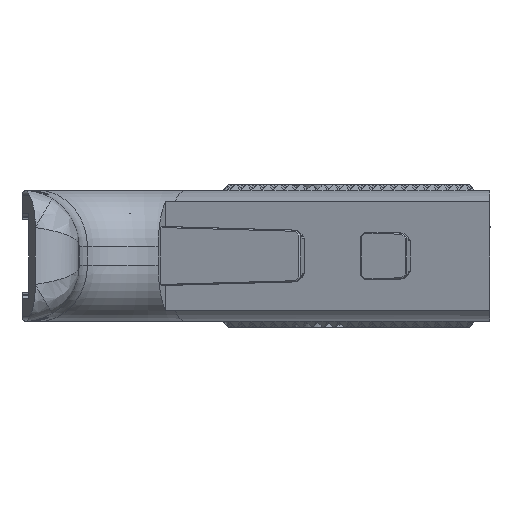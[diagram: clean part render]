
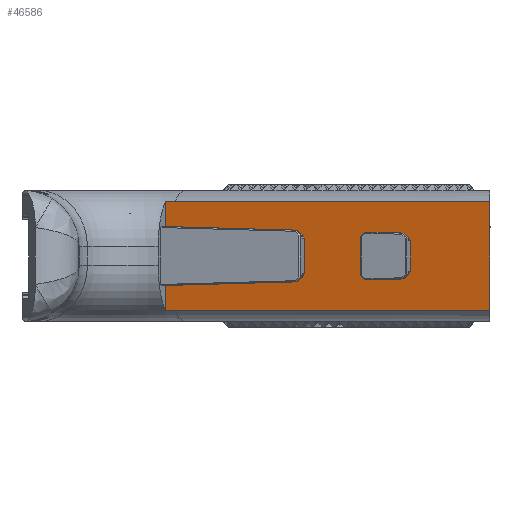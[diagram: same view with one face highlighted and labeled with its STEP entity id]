
A CAD part, left-side view. The second image highlights one B-rep face of the part: STEP entity #46586.
In plain terms, the highlighted planar face has unit normal (-0.951, 0.309, 0).
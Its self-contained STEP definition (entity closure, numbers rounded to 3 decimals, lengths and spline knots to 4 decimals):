
#2528=PLANE('',#49719);
#2773=FACE_BOUND('',#19868,.T.);
#7824=LINE('',#89198,#13351);
#7842=LINE('',#89236,#13369);
#7850=LINE('',#89253,#13377);
#7855=LINE('',#89262,#13382);
#7857=LINE('',#89265,#13384);
#7859=LINE('',#89270,#13386);
#7861=LINE('',#89274,#13388);
#7863=LINE('',#89277,#13390);
#7865=LINE('',#89281,#13392);
#7866=LINE('',#89283,#13393);
#7872=LINE('',#89296,#13399);
#7874=LINE('',#89300,#13401);
#7875=LINE('',#89303,#13402);
#7877=LINE('',#89307,#13404);
#7878=LINE('',#89317,#13405);
#7879=LINE('',#89319,#13406);
#7880=LINE('',#89321,#13407);
#7881=LINE('',#89331,#13408);
#7882=LINE('',#89332,#13409);
#13351=VECTOR('',#60471,0.3937);
#13369=VECTOR('',#60507,0.3937);
#13377=VECTOR('',#60521,0.3937);
#13382=VECTOR('',#60530,0.3937);
#13384=VECTOR('',#60534,0.3937);
#13386=VECTOR('',#60538,0.3937);
#13388=VECTOR('',#60542,0.3937);
#13390=VECTOR('',#60546,0.3937);
#13392=VECTOR('',#60550,0.3937);
#13393=VECTOR('',#60553,0.3937);
#13399=VECTOR('',#60569,0.3937);
#13401=VECTOR('',#60573,0.3937);
#13402=VECTOR('',#60576,0.3937);
#13404=VECTOR('',#60580,0.3937);
#13405=VECTOR('',#60581,0.3937);
#13406=VECTOR('',#60582,0.3937);
#13407=VECTOR('',#60583,0.3937);
#13408=VECTOR('',#60584,0.3937);
#13409=VECTOR('',#60585,0.3937);
#16849=FACE_OUTER_BOUND('',#19867,.T.);
#19867=EDGE_LOOP('',(#41645,#41646,#41647,#41648,#41649,#41650,#41651,#41652,
#41653,#41654,#41655,#41656));
#19868=EDGE_LOOP('',(#41657,#41658,#41659,#41660,#41661,#41662,#41663,#41664,
#41665));
#20883=B_SPLINE_CURVE_WITH_KNOTS('',3,(#89309,#89310,#89311,#89312,#89313,
#89314,#89315),.UNSPECIFIED.,.F.,.F.,(4,3,4),(0.,0.1181,0.2155),
 .UNSPECIFIED.);
#20884=B_SPLINE_CURVE_WITH_KNOTS('',3,(#89323,#89324,#89325,#89326,#89327,
#89328,#89329),.UNSPECIFIED.,.F.,.F.,(4,3,4),(-0.2155,-0.1181,
0.),.UNSPECIFIED.);
#23791=VERTEX_POINT('',#89195);
#23792=VERTEX_POINT('',#89197);
#23802=VERTEX_POINT('',#89233);
#23803=VERTEX_POINT('',#89235);
#23808=VERTEX_POINT('',#89250);
#23809=VERTEX_POINT('',#89252);
#23811=VERTEX_POINT('',#89261);
#23812=VERTEX_POINT('',#89267);
#23813=VERTEX_POINT('',#89269);
#23814=VERTEX_POINT('',#89273);
#23815=VERTEX_POINT('',#89279);
#23817=VERTEX_POINT('',#89294);
#23818=VERTEX_POINT('',#89298);
#23819=VERTEX_POINT('',#89302);
#23820=VERTEX_POINT('',#89306);
#23821=VERTEX_POINT('',#89308);
#23822=VERTEX_POINT('',#89316);
#23823=VERTEX_POINT('',#89318);
#23824=VERTEX_POINT('',#89320);
#23825=VERTEX_POINT('',#89322);
#23826=VERTEX_POINT('',#89330);
#29843=EDGE_CURVE('',#23792,#23791,#7824,.T.);
#29861=EDGE_CURVE('',#23802,#23803,#7842,.T.);
#29869=EDGE_CURVE('',#23808,#23809,#7850,.F.);
#29874=EDGE_CURVE('',#23792,#23811,#7855,.F.);
#29876=EDGE_CURVE('',#23808,#23811,#7857,.T.);
#29878=EDGE_CURVE('',#23812,#23813,#7859,.F.);
#29880=EDGE_CURVE('',#23814,#23813,#7861,.T.);
#29882=EDGE_CURVE('',#23812,#23809,#7863,.T.);
#29884=EDGE_CURVE('',#23815,#23791,#7865,.F.);
#29885=EDGE_CURVE('',#23814,#23815,#7866,.F.);
#29891=EDGE_CURVE('',#23817,#23802,#7872,.F.);
#29893=EDGE_CURVE('',#23817,#23818,#7874,.T.);
#29894=EDGE_CURVE('',#23803,#23819,#7875,.F.);
#29896=EDGE_CURVE('',#23820,#23818,#7877,.T.);
#29897=EDGE_CURVE('',#23821,#23820,#20883,.T.);
#29898=EDGE_CURVE('',#23822,#23821,#7878,.T.);
#29899=EDGE_CURVE('',#23823,#23822,#7879,.T.);
#29900=EDGE_CURVE('',#23824,#23823,#7880,.T.);
#29901=EDGE_CURVE('',#23825,#23824,#20884,.T.);
#29902=EDGE_CURVE('',#23826,#23825,#7881,.T.);
#29903=EDGE_CURVE('',#23826,#23819,#7882,.T.);
#41645=ORIENTED_EDGE('',*,*,#29893,.T.);
#41646=ORIENTED_EDGE('',*,*,#29896,.F.);
#41647=ORIENTED_EDGE('',*,*,#29897,.F.);
#41648=ORIENTED_EDGE('',*,*,#29898,.F.);
#41649=ORIENTED_EDGE('',*,*,#29899,.F.);
#41650=ORIENTED_EDGE('',*,*,#29900,.F.);
#41651=ORIENTED_EDGE('',*,*,#29901,.F.);
#41652=ORIENTED_EDGE('',*,*,#29902,.F.);
#41653=ORIENTED_EDGE('',*,*,#29903,.T.);
#41654=ORIENTED_EDGE('',*,*,#29894,.F.);
#41655=ORIENTED_EDGE('',*,*,#29861,.F.);
#41656=ORIENTED_EDGE('',*,*,#29891,.F.);
#41657=ORIENTED_EDGE('',*,*,#29843,.T.);
#41658=ORIENTED_EDGE('',*,*,#29884,.F.);
#41659=ORIENTED_EDGE('',*,*,#29885,.F.);
#41660=ORIENTED_EDGE('',*,*,#29880,.T.);
#41661=ORIENTED_EDGE('',*,*,#29878,.F.);
#41662=ORIENTED_EDGE('',*,*,#29882,.T.);
#41663=ORIENTED_EDGE('',*,*,#29869,.F.);
#41664=ORIENTED_EDGE('',*,*,#29876,.T.);
#41665=ORIENTED_EDGE('',*,*,#29874,.F.);
#46586=ADVANCED_FACE('',(#16849,#2773),#2528,.T.);
#49719=AXIS2_PLACEMENT_3D('',#89305,#60578,#60579);
#60471=DIRECTION('',(0.,0.,1.));
#60507=DIRECTION('',(0.,0.,1.));
#60521=DIRECTION('',(0.216,0.664,-0.716));
#60530=DIRECTION('',(0.221,0.681,0.698));
#60534=DIRECTION('',(0.309,0.951,-0.026));
#60538=DIRECTION('',(-0.216,-0.664,-0.716));
#60542=DIRECTION('',(-0.309,-0.951,-0.026));
#60546=DIRECTION('',(0.,0.,-1.));
#60550=DIRECTION('',(-0.12,-0.37,0.921));
#60553=DIRECTION('',(-0.221,-0.681,0.698));
#60569=DIRECTION('',(0.216,0.664,-0.716));
#60573=DIRECTION('',(0.309,0.951,-0.026));
#60576=DIRECTION('',(-0.216,-0.664,-0.716));
#60578=DIRECTION('center_axis',(-0.951,0.309,0.));
#60579=DIRECTION('ref_axis',(0.,0.,
1.));
#60580=DIRECTION('',(0.,0.,1.));
#60581=DIRECTION('',(0.309,0.951,0.));
#60582=DIRECTION('',(0.,0.,-1.));
#60583=DIRECTION('',(-0.309,-0.951,0.));
#60584=DIRECTION('',(0.,0.,1.));
#60585=DIRECTION('',(-0.309,-0.951,-0.026));
#89195=CARTESIAN_POINT('',(-2.8962,-0.8838,-0.6352));
#89197=CARTESIAN_POINT('',(-2.8962,-0.8838,-0.9101));
#89198=CARTESIAN_POINT('',(-2.8962,-0.8838,-0.7677));
#89233=CARTESIAN_POINT('',(-2.7262,-0.3607,-0.9245));
#89235=CARTESIAN_POINT('',(-2.7262,-0.3607,-0.6109));
#89236=CARTESIAN_POINT('',(-2.7262,-0.3607,-0.9154));
#89250=CARTESIAN_POINT('',(-3.0247,-1.2792,-0.909));
#89252=CARTESIAN_POINT('',(-3.0277,-1.2886,-0.8989));
#89253=CARTESIAN_POINT('',(-2.9908,-1.1749,-1.0217));
#89261=CARTESIAN_POINT('',(-2.8992,-0.8932,-0.9197));
#89262=CARTESIAN_POINT('',(-2.8709,-0.806,-0.8303));
#89265=CARTESIAN_POINT('',(-3.0469,-1.3476,-0.9072));
#89267=CARTESIAN_POINT('',(-3.0277,-1.2886,-0.6365));
#89269=CARTESIAN_POINT('',(-3.0247,-1.2792,-0.6264));
#89270=CARTESIAN_POINT('',(-2.9908,-1.1749,-0.5138));
#89273=CARTESIAN_POINT('',(-2.8992,-0.8932,-0.6158));
#89274=CARTESIAN_POINT('',(-3.0469,-1.3476,-0.6283));
#89277=CARTESIAN_POINT('',(-3.0277,-1.2886,-0.899));
#89279=CARTESIAN_POINT('',(-2.8984,-0.8905,-0.6185));
#89281=CARTESIAN_POINT('',(-2.885,-0.8493,-0.7213));
#89283=CARTESIAN_POINT('',(-2.8709,-0.806,-0.7051));
#89294=CARTESIAN_POINT('',(-2.7232,-0.3514,-0.9346));
#89296=CARTESIAN_POINT('',(-2.7647,-0.479,-0.7968));
#89298=CARTESIAN_POINT('',(-2.3324,0.8513,-0.9677));
#89300=CARTESIAN_POINT('',(-3.0469,-1.3476,-0.9072));
#89302=CARTESIAN_POINT('',(-2.7232,-0.3514,-0.6008));
#89303=CARTESIAN_POINT('',(-2.7647,-0.479,-0.7386));
#89305=CARTESIAN_POINT('Origin',(-2.8375,-0.7031,-0.7677));
#89306=CARTESIAN_POINT('',(-2.3324,0.8513,-1.2459));
#89307=CARTESIAN_POINT('',(-2.3324,0.8513,-1.0302));
#89308=CARTESIAN_POINT('',(-2.3592,0.7689,-1.2425));
#89309=CARTESIAN_POINT('Ctrl Pts',(-2.3592,0.7689,
-1.2425));
#89310=CARTESIAN_POINT('Ctrl Pts',(-2.3544,0.7836,
-1.2425));
#89311=CARTESIAN_POINT('Ctrl Pts',(-2.3495,0.7986,
-1.2428));
#89312=CARTESIAN_POINT('Ctrl Pts',(-2.3446,0.8138,
-1.2435));
#89313=CARTESIAN_POINT('Ctrl Pts',(-2.3405,0.8264,
-1.2441));
#89314=CARTESIAN_POINT('Ctrl Pts',(-2.3365,0.8388,
-1.2449));
#89315=CARTESIAN_POINT('Ctrl Pts',(-2.3324,0.8513,-1.2459));
#89316=CARTESIAN_POINT('',(-3.2516,-1.9775,-1.2425));
#89317=CARTESIAN_POINT('',(-2.1969,1.2684,-1.2425));
#89318=CARTESIAN_POINT('',(-3.2516,-1.9775,-0.2929));
#89319=CARTESIAN_POINT('',(-3.2516,-1.9775,-0.3839));
#89320=CARTESIAN_POINT('',(-2.3592,0.7689,-0.2929));
#89321=CARTESIAN_POINT('',(-2.6906,-0.2509,-0.2929));
#89322=CARTESIAN_POINT('',(-2.3324,0.8513,-0.2895));
#89323=CARTESIAN_POINT('Ctrl Pts',(-2.3324,0.8513,-0.2895));
#89324=CARTESIAN_POINT('Ctrl Pts',(-2.3365,0.8388,
-0.2905));
#89325=CARTESIAN_POINT('Ctrl Pts',(-2.3405,0.8264,
-0.2913));
#89326=CARTESIAN_POINT('Ctrl Pts',(-2.3446,0.8138,
-0.2919));
#89327=CARTESIAN_POINT('Ctrl Pts',(-2.3495,0.7986,
-0.2926));
#89328=CARTESIAN_POINT('Ctrl Pts',(-2.3544,0.7836,
-0.2929));
#89329=CARTESIAN_POINT('Ctrl Pts',(-2.3592,0.7689,
-0.2929));
#89330=CARTESIAN_POINT('',(-2.3324,0.8513,-0.5677));
#89331=CARTESIAN_POINT('',(-2.3324,0.8513,-0.7677));
#89332=CARTESIAN_POINT('',(-3.0469,-1.3476,-0.6283));
